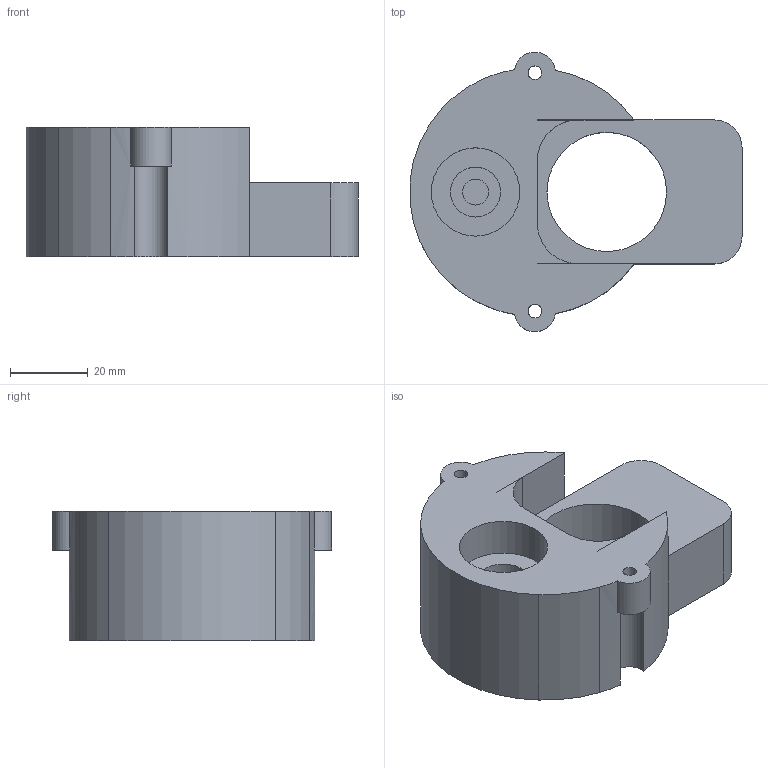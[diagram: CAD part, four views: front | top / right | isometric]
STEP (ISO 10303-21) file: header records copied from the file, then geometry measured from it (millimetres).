
FILE_DESCRIPTION(('FreeCAD Model'),'2;1');
FILE_NAME( 'mp-1 endcap.step', '2016-02-20T16:20:08',('Author'),(''), 'Open CASCADE STEP processor 6.8','FreeCAD','Unknown');
FILE_SCHEMA(('AUTOMOTIVE_DESIGN_CC2 { 1 2 10303 214 -1 1 5 4 }'));
Length unit declared in the file: millimetre
Products named in the file (1): Pocket019
Bounding box: 85.62 x 72.05 x 33.28 mm (x, y, z)
Volume: 87374.5 mm3; surface area: 20346.5 mm2
Topology: 1 solids, 1 shells, 57 faces, 154 edges, 101 vertices
Faces by surface type: plane 30, cylinder 27
Full cylindrical faces by diameter (mm): 3.5 x2, 6.7 x1, 12.9 x1, 22.8 x1
Entity records: 3973 total; most frequent: CARTESIAN_POINT 1082, DIRECTION 512, ORIENTED_EDGE 308, PCURVE 308, DEFINITIONAL_REPRESENTATION 308, LINE 204, VECTOR 204, EDGE_CURVE 154
